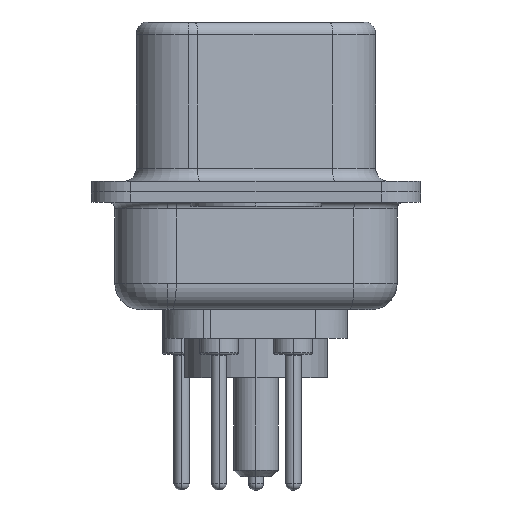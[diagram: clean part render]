
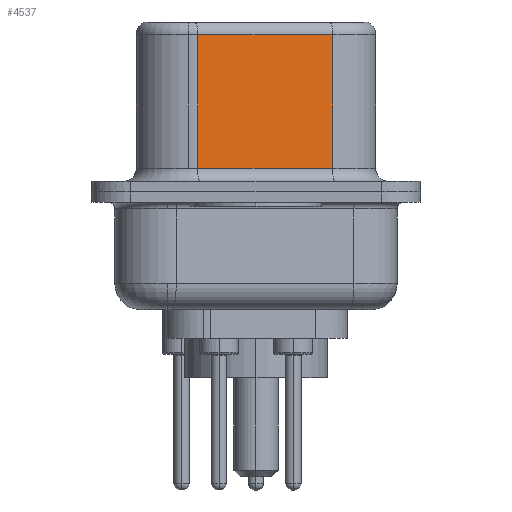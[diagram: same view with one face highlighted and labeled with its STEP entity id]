
A CAD part, left-side view. The second image highlights one B-rep face of the part: STEP entity #4537.
In plain terms, the highlighted planar face has unit normal (-0.985, -0.174, 0).
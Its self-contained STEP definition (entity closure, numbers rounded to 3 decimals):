
#261 = LINE ( 'NONE', #719, #10230 ) ;
#353 = CARTESIAN_POINT ( 'NONE',  ( 3.675, 2.233, 6.02 ) ) ;
#392 = ORIENTED_EDGE ( 'NONE', *, *, #4930, .F. ) ;
#560 = CARTESIAN_POINT ( 'NONE',  ( 4.585, -2.927, 6.52 ) ) ;
#624 = ORIENTED_EDGE ( 'NONE', *, *, #16483, .T. ) ;
#683 = DIRECTION ( 'NONE',  ( 0., 0., -1. ) ) ;
#719 = CARTESIAN_POINT ( 'NONE',  ( 4.585, -2.927, 6.02 ) ) ;
#2194 = VERTEX_POINT ( 'NONE', #353 ) ;
#3503 = EDGE_CURVE ( 'NONE', #2194, #5816, #13489, .T. ) ;
#3925 = CARTESIAN_POINT ( 'NONE',  ( 4.585, -2.927, 0.9 ) ) ;
#4537 = ADVANCED_FACE ( 'NONE', ( #5760 ), #15267, .F. ) ;
#4930 = EDGE_CURVE ( 'NONE', #18548, #5800, #14322, .T. ) ;
#5760 = FACE_OUTER_BOUND ( 'NONE', #16953, .T. ) ;
#5800 = VERTEX_POINT ( 'NONE', #3925 ) ;
#5816 = VERTEX_POINT ( 'NONE', #8381 ) ;
#6419 = VECTOR ( 'NONE', #683, 1000. ) ;
#6661 = DIRECTION ( 'NONE',  ( 0.985, 0.174, 0. ) ) ;
#8381 = CARTESIAN_POINT ( 'NONE',  ( 3.675, 2.233, 0.9 ) ) ;
#8740 = CARTESIAN_POINT ( 'NONE',  ( 4.585, -2.927, 6.02 ) ) ;
#8749 = EDGE_CURVE ( 'NONE', #18548, #2194, #261, .T. ) ;
#9519 = CARTESIAN_POINT ( 'NONE',  ( 4.585, -2.927, 6.52 ) ) ;
#9652 = VECTOR ( 'NONE', #10137, 1000. ) ;
#10065 = CARTESIAN_POINT ( 'NONE',  ( 3.675, 2.233, 6.52 ) ) ;
#10137 = DIRECTION ( 'NONE',  ( 0., 0., -1. ) ) ;
#10230 = VECTOR ( 'NONE', #10719, 1000. ) ;
#10719 = DIRECTION ( 'NONE',  ( -0.174, 0.985, 0. ) ) ;
#12631 = DIRECTION ( 'NONE',  ( -0.174, 0.985, 0. ) ) ;
#13489 = LINE ( 'NONE', #10065, #9652 ) ;
#13545 = LINE ( 'NONE', #15882, #16276 ) ;
#14322 = LINE ( 'NONE', #560, #6419 ) ;
#15267 = PLANE ( 'NONE',  #16288 ) ;
#15863 = ORIENTED_EDGE ( 'NONE', *, *, #3503, .T. ) ;
#15882 = CARTESIAN_POINT ( 'NONE',  ( 4.585, -2.927, 0.9 ) ) ;
#16110 = ORIENTED_EDGE ( 'NONE', *, *, #8749, .T. ) ;
#16276 = VECTOR ( 'NONE', #18631, 1000. ) ;
#16288 = AXIS2_PLACEMENT_3D ( 'NONE', #9519, #6661, #12631 ) ;
#16483 = EDGE_CURVE ( 'NONE', #5816, #5800, #13545, .T. ) ;
#16953 = EDGE_LOOP ( 'NONE', ( #392, #16110, #15863, #624 ) ) ;
#18548 = VERTEX_POINT ( 'NONE', #8740 ) ;
#18631 = DIRECTION ( 'NONE',  ( 0.174, -0.985, 0. ) ) ;
